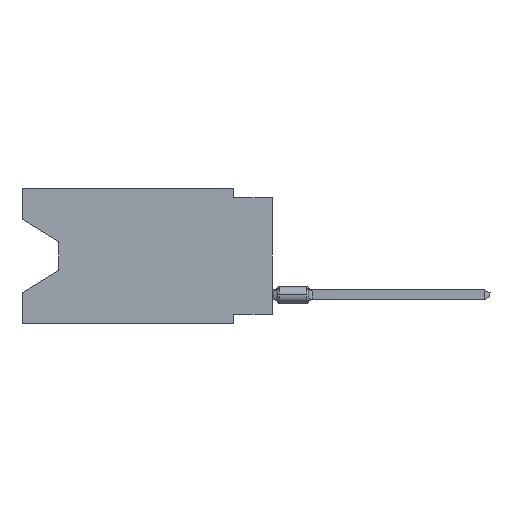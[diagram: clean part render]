
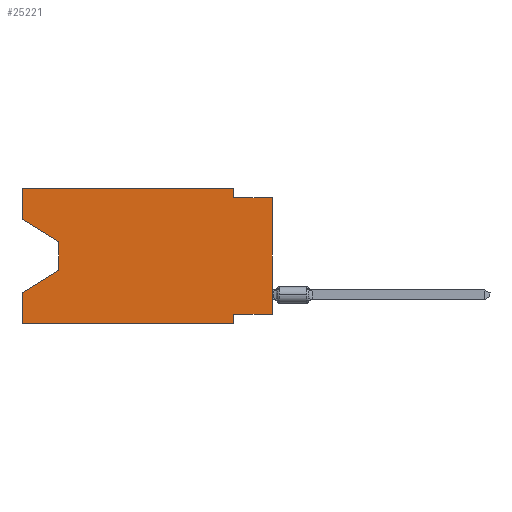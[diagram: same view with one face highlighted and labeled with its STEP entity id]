
A CAD part, left-side view. The second image highlights one B-rep face of the part: STEP entity #25221.
In plain terms, the highlighted planar face has unit normal (-1, 0, 0).
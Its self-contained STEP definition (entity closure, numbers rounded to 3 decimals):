
#1667 = VERTEX_POINT ( 'NONE', #55521 ) ;
#2609 = VECTOR ( 'NONE', #36034, 1000. ) ;
#2724 = VECTOR ( 'NONE', #9725, 1000. ) ;
#5228 = DIRECTION ( 'NONE',  ( 0., -1., 0. ) ) ;
#5727 = LINE ( 'NONE', #38376, #29889 ) ;
#6604 = CARTESIAN_POINT ( 'NONE',  ( 0., 16.383, -6.852 ) ) ;
#7757 = CARTESIAN_POINT ( 'NONE',  ( 0., 16.383, 0. ) ) ;
#8277 = VERTEX_POINT ( 'NONE', #55715 ) ;
#8571 = ORIENTED_EDGE ( 'NONE', *, *, #68019, .F. ) ;
#9104 = EDGE_LOOP ( 'NONE', ( #60198, #78228, #55292, #29693, #62135, #37113, #12738, #83649, #43534, #25456, #8571, #81022 ) ) ;
#9444 = VERTEX_POINT ( 'NONE', #6604 ) ;
#9725 = DIRECTION ( 'NONE',  ( 0., 0., -1. ) ) ;
#10328 = VECTOR ( 'NONE', #26587, 1000. ) ;
#10351 = VERTEX_POINT ( 'NONE', #83218 ) ;
#11486 = LINE ( 'NONE', #24982, #35035 ) ;
#11746 = LINE ( 'NONE', #64820, #57463 ) ;
#12443 = EDGE_CURVE ( 'NONE', #56121, #83607, #82131, .T. ) ;
#12738 = ORIENTED_EDGE ( 'NONE', *, *, #44973, .F. ) ;
#14177 = CARTESIAN_POINT ( 'NONE',  ( 0., 0., -8.255 ) ) ;
#15110 = VECTOR ( 'NONE', #48227, 1000. ) ;
#16381 = CARTESIAN_POINT ( 'NONE',  ( 0., 13.97, -3.505 ) ) ;
#16426 = VECTOR ( 'NONE', #58993, 1000. ) ;
#17163 = DIRECTION ( 'NONE',  ( 0., -1., 0. ) ) ;
#17276 = LINE ( 'NONE', #43838, #2609 ) ;
#17809 = EDGE_CURVE ( 'NONE', #1667, #8277, #11746, .T. ) ;
#17811 = CARTESIAN_POINT ( 'NONE',  ( 0., 2.54, -0.635 ) ) ;
#19737 = EDGE_CURVE ( 'NONE', #84640, #49485, #36404, .T. ) ;
#20054 = LINE ( 'NONE', #46601, #10328 ) ;
#21693 = DIRECTION ( 'NONE',  ( 0., 0., 1. ) ) ;
#22130 = VERTEX_POINT ( 'NONE', #71256 ) ;
#23758 = VERTEX_POINT ( 'NONE', #25176 ) ;
#24881 = VECTOR ( 'NONE', #21693, 1000. ) ;
#24982 = CARTESIAN_POINT ( 'NONE',  ( 0., 0., -0.635 ) ) ;
#25176 = CARTESIAN_POINT ( 'NONE',  ( 0., 16.383, -2.038 ) ) ;
#25221 = ADVANCED_FACE ( 'NONE', ( #81703 ), #28636, .F. ) ;
#25265 = EDGE_CURVE ( 'NONE', #1667, #9444, #54737, .T. ) ;
#25395 = EDGE_CURVE ( 'NONE', #22130, #37559, #17276, .T. ) ;
#25456 = ORIENTED_EDGE ( 'NONE', *, *, #25395, .F. ) ;
#26587 = DIRECTION ( 'NONE',  ( 0., 0., 1. ) ) ;
#28205 = DIRECTION ( 'NONE',  ( 0., 0., -1. ) ) ;
#28636 = PLANE ( 'NONE',  #62368 ) ;
#29693 = ORIENTED_EDGE ( 'NONE', *, *, #25265, .F. ) ;
#29889 = VECTOR ( 'NONE', #57504, 1000. ) ;
#34321 = DIRECTION ( 'NONE',  ( 1., 0., 0. ) ) ;
#35035 = VECTOR ( 'NONE', #17163, 1000. ) ;
#36034 = DIRECTION ( 'NONE',  ( 0., 0., -1. ) ) ;
#36404 = LINE ( 'NONE', #16381, #52124 ) ;
#37113 = ORIENTED_EDGE ( 'NONE', *, *, #74517, .F. ) ;
#37559 = VERTEX_POINT ( 'NONE', #17811 ) ;
#38376 = CARTESIAN_POINT ( 'NONE',  ( 0., 16.383, 0. ) ) ;
#39433 = LINE ( 'NONE', #57710, #16426 ) ;
#43534 = ORIENTED_EDGE ( 'NONE', *, *, #49512, .F. ) ;
#43838 = CARTESIAN_POINT ( 'NONE',  ( 0., 2.54, 0. ) ) ;
#44973 = EDGE_CURVE ( 'NONE', #56121, #10351, #39433, .T. ) ;
#45037 = CARTESIAN_POINT ( 'NONE',  ( 0., 13.97, -3.505 ) ) ;
#46601 = CARTESIAN_POINT ( 'NONE',  ( 0., 16.383, 0. ) ) ;
#48227 = DIRECTION ( 'NONE',  ( 0., 0., 1. ) ) ;
#49021 = DIRECTION ( 'NONE',  ( 0., 0., -1. ) ) ;
#49485 = VERTEX_POINT ( 'NONE', #84560 ) ;
#49512 = EDGE_CURVE ( 'NONE', #37559, #83607, #11486, .T. ) ;
#51745 = VECTOR ( 'NONE', #82099, 1000. ) ;
#52124 = VECTOR ( 'NONE', #49021, 1000. ) ;
#52180 = EDGE_CURVE ( 'NONE', #49485, #9444, #68795, .T. ) ;
#54737 = LINE ( 'NONE', #81268, #15110 ) ;
#55292 = ORIENTED_EDGE ( 'NONE', *, *, #52180, .T. ) ;
#55521 = CARTESIAN_POINT ( 'NONE',  ( 0., 16.383, -8.89 ) ) ;
#55715 = CARTESIAN_POINT ( 'NONE',  ( 0., 2.54, -8.89 ) ) ;
#55828 = CARTESIAN_POINT ( 'NONE',  ( 0., 2.54, -8.89 ) ) ;
#56121 = VERTEX_POINT ( 'NONE', #14177 ) ;
#57463 = VECTOR ( 'NONE', #5228, 1000. ) ;
#57504 = DIRECTION ( 'NONE',  ( 0., -1., 0. ) ) ;
#57710 = CARTESIAN_POINT ( 'NONE',  ( 0., 0., -8.255 ) ) ;
#58993 = DIRECTION ( 'NONE',  ( 0., 1., 0. ) ) ;
#60198 = ORIENTED_EDGE ( 'NONE', *, *, #60888, .T. ) ;
#60888 = EDGE_CURVE ( 'NONE', #23758, #84640, #75574, .T. ) ;
#61600 = CARTESIAN_POINT ( 'NONE',  ( 0., 0., -0.635 ) ) ;
#62135 = ORIENTED_EDGE ( 'NONE', *, *, #17809, .T. ) ;
#62284 = CARTESIAN_POINT ( 'NONE',  ( 0., 13.97, -5.385 ) ) ;
#62363 = LINE ( 'NONE', #55828, #2724 ) ;
#62368 = AXIS2_PLACEMENT_3D ( 'NONE', #7757, #34321, #28205 ) ;
#64820 = CARTESIAN_POINT ( 'NONE',  ( 0., 16.383, -8.89 ) ) ;
#66865 = EDGE_CURVE ( 'NONE', #23758, #78904, #20054, .T. ) ;
#68019 = EDGE_CURVE ( 'NONE', #78904, #22130, #5727, .T. ) ;
#68603 = CARTESIAN_POINT ( 'NONE',  ( 0., 16.383, -2.038 ) ) ;
#68795 = LINE ( 'NONE', #62284, #85046 ) ;
#71256 = CARTESIAN_POINT ( 'NONE',  ( 0., 2.54, 0. ) ) ;
#73882 = CARTESIAN_POINT ( 'NONE',  ( 0., 0., 0. ) ) ;
#74517 = EDGE_CURVE ( 'NONE', #10351, #8277, #62363, .T. ) ;
#75574 = LINE ( 'NONE', #68603, #51745 ) ;
#75767 = DIRECTION ( 'NONE',  ( 0., 0.855, -0.519 ) ) ;
#78228 = ORIENTED_EDGE ( 'NONE', *, *, #19737, .T. ) ;
#78904 = VERTEX_POINT ( 'NONE', #82525 ) ;
#81022 = ORIENTED_EDGE ( 'NONE', *, *, #66865, .F. ) ;
#81268 = CARTESIAN_POINT ( 'NONE',  ( 0., 16.383, 0. ) ) ;
#81703 = FACE_OUTER_BOUND ( 'NONE', #9104, .T. ) ;
#82099 = DIRECTION ( 'NONE',  ( 0., -0.855, -0.519 ) ) ;
#82131 = LINE ( 'NONE', #73882, #24881 ) ;
#82525 = CARTESIAN_POINT ( 'NONE',  ( 0., 16.383, 0. ) ) ;
#83218 = CARTESIAN_POINT ( 'NONE',  ( 0., 2.54, -8.255 ) ) ;
#83607 = VERTEX_POINT ( 'NONE', #61600 ) ;
#83649 = ORIENTED_EDGE ( 'NONE', *, *, #12443, .T. ) ;
#84560 = CARTESIAN_POINT ( 'NONE',  ( 0., 13.97, -5.385 ) ) ;
#84640 = VERTEX_POINT ( 'NONE', #45037 ) ;
#85046 = VECTOR ( 'NONE', #75767, 1000. ) ;
